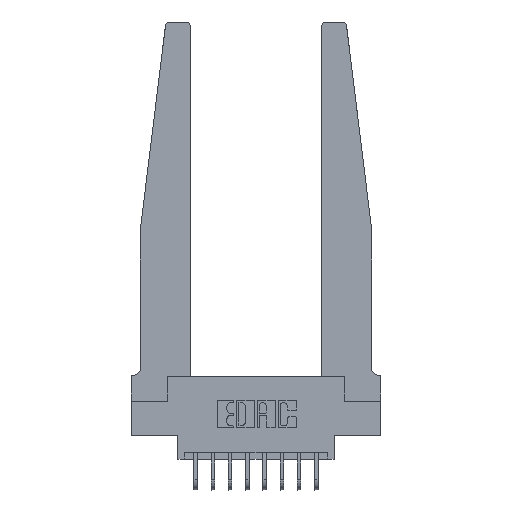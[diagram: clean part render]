
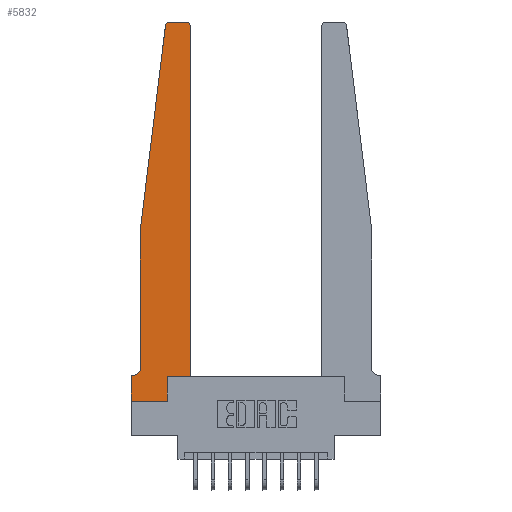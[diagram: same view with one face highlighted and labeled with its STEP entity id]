
A CAD part, top view. The second image highlights one B-rep face of the part: STEP entity #5832.
In plain terms, the highlighted planar face has unit normal (0, 0, 1).
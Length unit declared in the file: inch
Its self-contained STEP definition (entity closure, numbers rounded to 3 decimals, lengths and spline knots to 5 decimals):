
#529 = LINE ( 'NONE', #768, #8862 ) ;
#642 = CIRCLE ( 'NONE', #14895, 0.03 ) ;
#702 = EDGE_CURVE ( 'NONE', #9923, #11597, #6596, .T. ) ;
#768 = CARTESIAN_POINT ( 'NONE',  ( 0., 0., 0.37 ) ) ;
#901 = DIRECTION ( 'NONE',  ( 0., 0., 1. ) ) ;
#915 = FACE_OUTER_BOUND ( 'NONE', #15818, .T. ) ;
#1166 = VERTEX_POINT ( 'NONE', #15765 ) ;
#1349 = DIRECTION ( 'NONE',  ( -0.122, -0.992, 0. ) ) ;
#1555 = EDGE_CURVE ( 'NONE', #16208, #2966, #15915, .T. ) ;
#1703 = DIRECTION ( 'NONE',  ( 0., -1., 0. ) ) ;
#1880 = DIRECTION ( 'NONE',  ( -1., 0., 0. ) ) ;
#2115 = ORIENTED_EDGE ( 'NONE', *, *, #13254, .T. ) ;
#2349 = CARTESIAN_POINT ( 'NONE',  ( 0.425, 0.18, 0.37 ) ) ;
#2355 = CARTESIAN_POINT ( 'NONE',  ( 0.2605, 0., 0.37 ) ) ;
#2527 = DIRECTION ( 'NONE',  ( 0., 0., 1. ) ) ;
#2788 = AXIS2_PLACEMENT_3D ( 'NONE', #8906, #2527, #6654 ) ;
#2868 = CARTESIAN_POINT ( 'NONE',  ( 0.015, 0.1875, 0.37 ) ) ;
#2917 = LINE ( 'NONE', #12060, #7188 ) ;
#2966 = VERTEX_POINT ( 'NONE', #12947 ) ;
#2986 = CARTESIAN_POINT ( 'NONE',  ( 0., 0., 0.37 ) ) ;
#3107 = VERTEX_POINT ( 'NONE', #5552 ) ;
#3222 = VERTEX_POINT ( 'NONE', #5835 ) ;
#3478 = ORIENTED_EDGE ( 'NONE', *, *, #3866, .T. ) ;
#3491 = CARTESIAN_POINT ( 'NONE',  ( 0.395, 2.75, 0.37 ) ) ;
#3498 = EDGE_CURVE ( 'NONE', #13345, #6016, #8278, .T. ) ;
#3681 = CARTESIAN_POINT ( 'NONE',  ( 0.25, 2.75, 0.37 ) ) ;
#3866 = EDGE_CURVE ( 'NONE', #6016, #6870, #6240, .T. ) ;
#3886 = ORIENTED_EDGE ( 'NONE', *, *, #7599, .T. ) ;
#4362 = LINE ( 'NONE', #2986, #13065 ) ;
#4451 = LINE ( 'NONE', #5228, #5217 ) ;
#5217 = VECTOR ( 'NONE', #1349, 39.37008 ) ;
#5228 = CARTESIAN_POINT ( 'NONE',  ( 0.065, 1.25, 0.37 ) ) ;
#5552 = CARTESIAN_POINT ( 'NONE',  ( 0.065, 1.25, 0.37 ) ) ;
#5673 = CARTESIAN_POINT ( 'NONE',  ( 0.2605, 0.18, 0.37 ) ) ;
#5737 = EDGE_CURVE ( 'NONE', #6870, #3222, #11533, .T. ) ;
#5832 = ADVANCED_FACE ( 'NONE', ( #915 ), #10484, .T. ) ;
#5835 = CARTESIAN_POINT ( 'NONE',  ( 0.425, 2.72, 0.37 ) ) ;
#6016 = VERTEX_POINT ( 'NONE', #5673 ) ;
#6043 = ORIENTED_EDGE ( 'NONE', *, *, #14265, .T. ) ;
#6046 = CARTESIAN_POINT ( 'NONE',  ( 0.2605, 0.18, 0.37 ) ) ;
#6076 = ORIENTED_EDGE ( 'NONE', *, *, #702, .T. ) ;
#6233 = ORIENTED_EDGE ( 'NONE', *, *, #9486, .T. ) ;
#6240 = LINE ( 'NONE', #6321, #16019 ) ;
#6321 = CARTESIAN_POINT ( 'NONE',  ( 0.425, 0.18, 0.37 ) ) ;
#6500 = ORIENTED_EDGE ( 'NONE', *, *, #6987, .T. ) ;
#6568 = VECTOR ( 'NONE', #1880, 39.37008 ) ;
#6596 = CIRCLE ( 'NONE', #14246, 0.05 ) ;
#6654 = DIRECTION ( 'NONE',  ( 1., 0., 0. ) ) ;
#6870 = VERTEX_POINT ( 'NONE', #2349 ) ;
#6987 = EDGE_CURVE ( 'NONE', #1166, #9156, #529, .T. ) ;
#7014 = VECTOR ( 'NONE', #11374, 39.37008 ) ;
#7188 = VECTOR ( 'NONE', #1703, 39.37008 ) ;
#7283 = DIRECTION ( 'NONE',  ( 0., -1., 0. ) ) ;
#7346 = ORIENTED_EDGE ( 'NONE', *, *, #10778, .T. ) ;
#7599 = EDGE_CURVE ( 'NONE', #3222, #14611, #642, .T. ) ;
#8278 = LINE ( 'NONE', #6046, #12996 ) ;
#8862 = VECTOR ( 'NONE', #7283, 39.37008 ) ;
#8906 = CARTESIAN_POINT ( 'NONE',  ( 0.27653, 2.72, 0.37 ) ) ;
#9076 = EDGE_CURVE ( 'NONE', #11597, #1166, #10907, .T. ) ;
#9156 = VERTEX_POINT ( 'NONE', #9700 ) ;
#9225 = AXIS2_PLACEMENT_3D ( 'NONE', #14426, #16896, #14513 ) ;
#9340 = CARTESIAN_POINT ( 'NONE',  ( 0.27653, 2.75, 0.37 ) ) ;
#9486 = EDGE_CURVE ( 'NONE', #2966, #3107, #4451, .T. ) ;
#9700 = CARTESIAN_POINT ( 'NONE',  ( 0., 0., 0.37 ) ) ;
#9923 = VERTEX_POINT ( 'NONE', #14551 ) ;
#10378 = LINE ( 'NONE', #3681, #14521 ) ;
#10484 = PLANE ( 'NONE',  #9225 ) ;
#10778 = EDGE_CURVE ( 'NONE', #9156, #13345, #4362, .T. ) ;
#10907 = LINE ( 'NONE', #12242, #6568 ) ;
#11188 = CARTESIAN_POINT ( 'NONE',  ( 0.015, 0.2375, 0.37 ) ) ;
#11374 = DIRECTION ( 'NONE',  ( 0., 1., 0. ) ) ;
#11533 = LINE ( 'NONE', #15132, #7014 ) ;
#11597 = VERTEX_POINT ( 'NONE', #2868 ) ;
#12060 = CARTESIAN_POINT ( 'NONE',  ( 0.065, 1.25, 0.37 ) ) ;
#12187 = DIRECTION ( 'NONE',  ( 0., 1., 0. ) ) ;
#12242 = CARTESIAN_POINT ( 'NONE',  ( 0.065, 0.1875, 0.37 ) ) ;
#12347 = ORIENTED_EDGE ( 'NONE', *, *, #1555, .T. ) ;
#12947 = CARTESIAN_POINT ( 'NONE',  ( 0.24675, 2.72367, 0.37 ) ) ;
#12996 = VECTOR ( 'NONE', #12187, 39.37008 ) ;
#13065 = VECTOR ( 'NONE', #13428, 39.37008 ) ;
#13250 = ORIENTED_EDGE ( 'NONE', *, *, #9076, .T. ) ;
#13254 = EDGE_CURVE ( 'NONE', #3107, #9923, #2917, .T. ) ;
#13345 = VERTEX_POINT ( 'NONE', #2355 ) ;
#13428 = DIRECTION ( 'NONE',  ( 1., 0., 0. ) ) ;
#13561 = DIRECTION ( 'NONE',  ( 0., 0., -1. ) ) ;
#14095 = ORIENTED_EDGE ( 'NONE', *, *, #3498, .T. ) ;
#14246 = AXIS2_PLACEMENT_3D ( 'NONE', #11188, #13561, #14795 ) ;
#14265 = EDGE_CURVE ( 'NONE', #14611, #16208, #10378, .T. ) ;
#14426 = CARTESIAN_POINT ( 'NONE',  ( 0., 0.1875, 0.37 ) ) ;
#14513 = DIRECTION ( 'NONE',  ( 1., 0., 0. ) ) ;
#14521 = VECTOR ( 'NONE', #15579, 39.37008 ) ;
#14551 = CARTESIAN_POINT ( 'NONE',  ( 0.065, 0.2375, 0.37 ) ) ;
#14611 = VERTEX_POINT ( 'NONE', #3491 ) ;
#14795 = DIRECTION ( 'NONE',  ( -1., 0., 0. ) ) ;
#14895 = AXIS2_PLACEMENT_3D ( 'NONE', #16564, #901, #15275 ) ;
#15132 = CARTESIAN_POINT ( 'NONE',  ( 0.425, 0.18, 0.37 ) ) ;
#15275 = DIRECTION ( 'NONE',  ( 1., 0., 0. ) ) ;
#15579 = DIRECTION ( 'NONE',  ( -1., 0., 0. ) ) ;
#15607 = ORIENTED_EDGE ( 'NONE', *, *, #5737, .T. ) ;
#15765 = CARTESIAN_POINT ( 'NONE',  ( 0., 0.1875, 0.37 ) ) ;
#15818 = EDGE_LOOP ( 'NONE', ( #6043, #12347, #6233, #2115, #6076, #13250, #6500, #7346, #14095, #3478, #15607, #3886 ) ) ;
#15915 = CIRCLE ( 'NONE', #2788, 0.03 ) ;
#16019 = VECTOR ( 'NONE', #16734, 39.37008 ) ;
#16208 = VERTEX_POINT ( 'NONE', #9340 ) ;
#16564 = CARTESIAN_POINT ( 'NONE',  ( 0.395, 2.72, 0.37 ) ) ;
#16734 = DIRECTION ( 'NONE',  ( 1., 0., 0. ) ) ;
#16896 = DIRECTION ( 'NONE',  ( 0., 0., 1. ) ) ;
